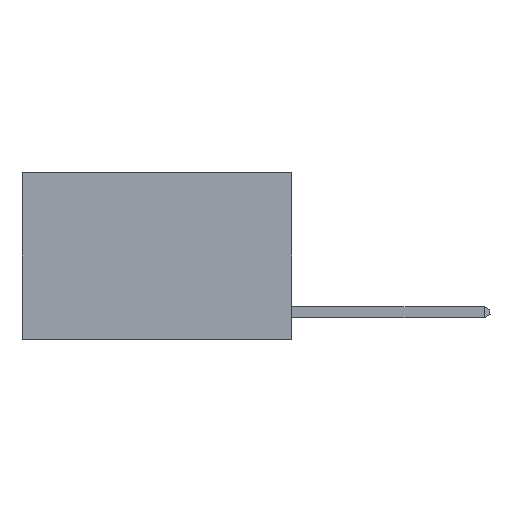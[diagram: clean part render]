
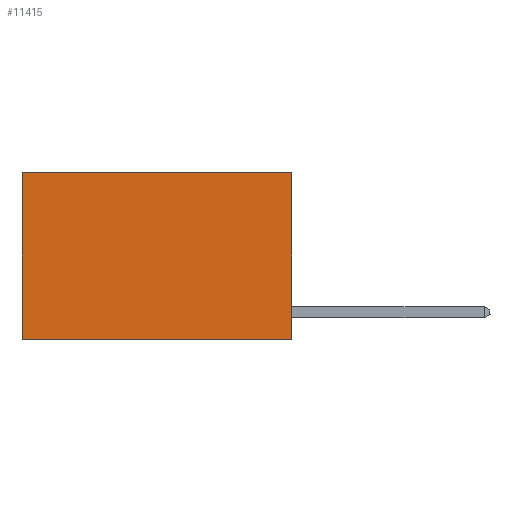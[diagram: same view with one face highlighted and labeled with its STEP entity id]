
A CAD part, left-side view. The second image highlights one B-rep face of the part: STEP entity #11415.
In plain terms, the highlighted planar face has unit normal (-1, 0, 0).
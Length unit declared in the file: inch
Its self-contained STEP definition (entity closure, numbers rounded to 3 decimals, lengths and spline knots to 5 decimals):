
#355 = CARTESIAN_POINT ( 'NONE',  ( 0.2625, 0., 0. ) ) ;
#885 = LINE ( 'NONE', #10464, #4162 ) ;
#1100 = CARTESIAN_POINT ( 'NONE',  ( 0.2625, 0.6, 0. ) ) ;
#1175 = CARTESIAN_POINT ( 'NONE',  ( 0.2625, 0., 0. ) ) ;
#3240 = CARTESIAN_POINT ( 'NONE',  ( 0.2625, 0., -0.37 ) ) ;
#3653 = ORIENTED_EDGE ( 'NONE', *, *, #10262, .T. ) ;
#3892 = LINE ( 'NONE', #355, #4407 ) ;
#4162 = VECTOR ( 'NONE', #7942, 39.37008 ) ;
#4336 = ORIENTED_EDGE ( 'NONE', *, *, #9517, .F. ) ;
#4407 = VECTOR ( 'NONE', #12404, 39.37008 ) ;
#4417 = ORIENTED_EDGE ( 'NONE', *, *, #10564, .T. ) ;
#5788 = VECTOR ( 'NONE', #13451, 39.37008 ) ;
#6722 = LINE ( 'NONE', #14963, #8867 ) ;
#7293 = FACE_OUTER_BOUND ( 'NONE', #13561, .T. ) ;
#7942 = DIRECTION ( 'NONE',  ( 0., 0., -1. ) ) ;
#8070 = VERTEX_POINT ( 'NONE', #3240 ) ;
#8867 = VECTOR ( 'NONE', #10420, 39.37008 ) ;
#9517 = EDGE_CURVE ( 'NONE', #13416, #8070, #885, .T. ) ;
#10180 = ORIENTED_EDGE ( 'NONE', *, *, #14903, .F. ) ;
#10262 = EDGE_CURVE ( 'NONE', #11383, #12041, #6722, .T. ) ;
#10420 = DIRECTION ( 'NONE',  ( 0., 0., -1. ) ) ;
#10464 = CARTESIAN_POINT ( 'NONE',  ( 0.2625, 0., 0. ) ) ;
#10564 = EDGE_CURVE ( 'NONE', #13416, #11383, #3892, .T. ) ;
#11328 = CARTESIAN_POINT ( 'NONE',  ( 0.2625, 0., 0. ) ) ;
#11383 = VERTEX_POINT ( 'NONE', #1100 ) ;
#11415 = ADVANCED_FACE ( 'NONE', ( #7293 ), #15190, .F. ) ;
#12041 = VERTEX_POINT ( 'NONE', #15189 ) ;
#12093 = CARTESIAN_POINT ( 'NONE',  ( 0.2625, 0., -0.37 ) ) ;
#12404 = DIRECTION ( 'NONE',  ( 0., 1., 0. ) ) ;
#12416 = LINE ( 'NONE', #12093, #5788 ) ;
#13416 = VERTEX_POINT ( 'NONE', #11328 ) ;
#13451 = DIRECTION ( 'NONE',  ( 0., 1., 0. ) ) ;
#13561 = EDGE_LOOP ( 'NONE', ( #3653, #10180, #4336, #4417 ) ) ;
#13956 = AXIS2_PLACEMENT_3D ( 'NONE', #1175, #14586, #14741 ) ;
#14586 = DIRECTION ( 'NONE',  ( 1., 0., 0. ) ) ;
#14741 = DIRECTION ( 'NONE',  ( 0., 0., -1. ) ) ;
#14903 = EDGE_CURVE ( 'NONE', #8070, #12041, #12416, .T. ) ;
#14963 = CARTESIAN_POINT ( 'NONE',  ( 0.2625, 0.6, 0. ) ) ;
#15189 = CARTESIAN_POINT ( 'NONE',  ( 0.2625, 0.6, -0.37 ) ) ;
#15190 = PLANE ( 'NONE',  #13956 ) ;
